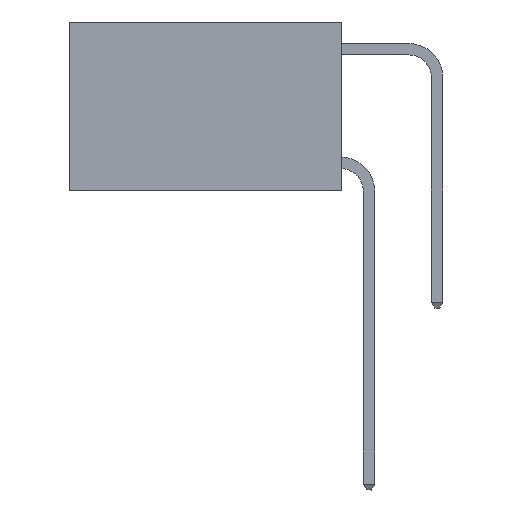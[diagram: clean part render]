
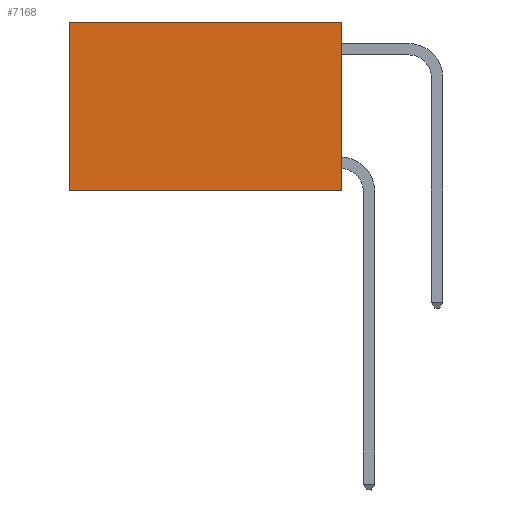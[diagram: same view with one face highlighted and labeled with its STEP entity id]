
A CAD part, left-side view. The second image highlights one B-rep face of the part: STEP entity #7168.
In plain terms, the highlighted planar face has unit normal (-1, 0, 0).
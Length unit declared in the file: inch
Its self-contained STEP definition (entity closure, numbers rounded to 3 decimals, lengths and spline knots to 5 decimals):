
#356 = DIRECTION ( 'NONE',  ( 0., 0., -1. ) ) ;
#441 = ORIENTED_EDGE ( 'NONE', *, *, #2513, .T. ) ;
#444 = CARTESIAN_POINT ( 'NONE',  ( 0.2625, 0., 0. ) ) ;
#667 = CARTESIAN_POINT ( 'NONE',  ( 0.2625, 0., -0.37 ) ) ;
#828 = VECTOR ( 'NONE', #6363, 39.37008 ) ;
#1103 = EDGE_LOOP ( 'NONE', ( #441, #8339, #7554, #8728 ) ) ;
#1671 = EDGE_CURVE ( 'NONE', #7377, #2193, #6111, .T. ) ;
#2081 = LINE ( 'NONE', #11866, #4154 ) ;
#2193 = VERTEX_POINT ( 'NONE', #9638 ) ;
#2513 = EDGE_CURVE ( 'NONE', #11694, #2193, #2081, .T. ) ;
#2599 = PLANE ( 'NONE',  #12122 ) ;
#3606 = DIRECTION ( 'NONE',  ( 0., 0., -1. ) ) ;
#3618 = LINE ( 'NONE', #5330, #828 ) ;
#3651 = FACE_OUTER_BOUND ( 'NONE', #1103, .T. ) ;
#3810 = CARTESIAN_POINT ( 'NONE',  ( 0.2625, 0.6, 0. ) ) ;
#4101 = EDGE_CURVE ( 'NONE', #6327, #11694, #3618, .T. ) ;
#4154 = VECTOR ( 'NONE', #9170, 39.37008 ) ;
#5330 = CARTESIAN_POINT ( 'NONE',  ( 0.2625, 0., 0. ) ) ;
#6111 = LINE ( 'NONE', #10835, #8871 ) ;
#6327 = VERTEX_POINT ( 'NONE', #7498 ) ;
#6363 = DIRECTION ( 'NONE',  ( 0., 1., 0. ) ) ;
#6399 = EDGE_CURVE ( 'NONE', #6327, #7377, #7712, .T. ) ;
#7168 = ADVANCED_FACE ( 'NONE', ( #3651 ), #2599, .F. ) ;
#7377 = VERTEX_POINT ( 'NONE', #667 ) ;
#7498 = CARTESIAN_POINT ( 'NONE',  ( 0.2625, 0., 0. ) ) ;
#7554 = ORIENTED_EDGE ( 'NONE', *, *, #6399, .F. ) ;
#7712 = LINE ( 'NONE', #444, #11419 ) ;
#8339 = ORIENTED_EDGE ( 'NONE', *, *, #1671, .F. ) ;
#8728 = ORIENTED_EDGE ( 'NONE', *, *, #4101, .T. ) ;
#8871 = VECTOR ( 'NONE', #10831, 39.37008 ) ;
#9170 = DIRECTION ( 'NONE',  ( 0., 0., -1. ) ) ;
#9425 = DIRECTION ( 'NONE',  ( 1., 0., 0. ) ) ;
#9638 = CARTESIAN_POINT ( 'NONE',  ( 0.2625, 0.6, -0.37 ) ) ;
#10831 = DIRECTION ( 'NONE',  ( 0., 1., 0. ) ) ;
#10835 = CARTESIAN_POINT ( 'NONE',  ( 0.2625, 0., -0.37 ) ) ;
#11419 = VECTOR ( 'NONE', #356, 39.37008 ) ;
#11694 = VERTEX_POINT ( 'NONE', #3810 ) ;
#11866 = CARTESIAN_POINT ( 'NONE',  ( 0.2625, 0.6, 0. ) ) ;
#12088 = CARTESIAN_POINT ( 'NONE',  ( 0.2625, 0., 0. ) ) ;
#12122 = AXIS2_PLACEMENT_3D ( 'NONE', #12088, #9425, #3606 ) ;
